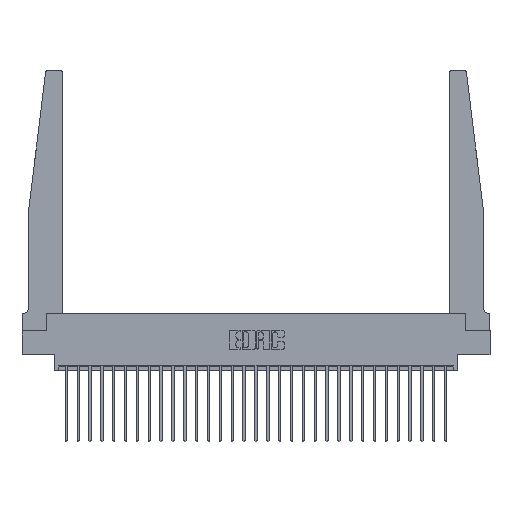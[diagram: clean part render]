
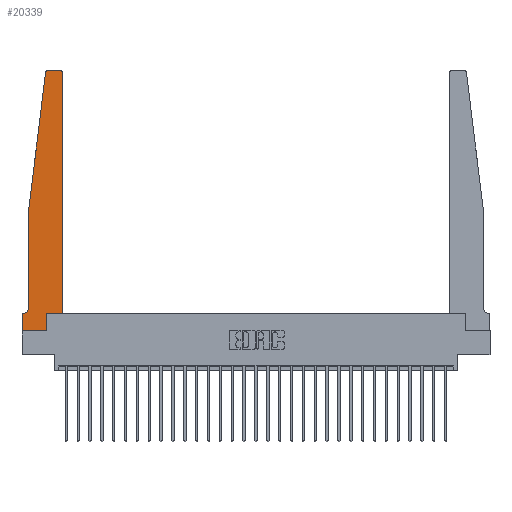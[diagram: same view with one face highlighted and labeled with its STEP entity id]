
A CAD part, top view. The second image highlights one B-rep face of the part: STEP entity #20339.
In plain terms, the highlighted planar face has unit normal (0, 0, 1).
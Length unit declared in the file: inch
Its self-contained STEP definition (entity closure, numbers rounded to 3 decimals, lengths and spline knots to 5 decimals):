
#234 = CIRCLE ( 'NONE', #23782, 0.03 ) ;
#404 = VECTOR ( 'NONE', #4082, 39.37008 ) ;
#507 = EDGE_CURVE ( 'NONE', #5747, #3042, #14602, .T. ) ;
#906 = FACE_OUTER_BOUND ( 'NONE', #13139, .T. ) ;
#1061 = CARTESIAN_POINT ( 'NONE',  ( 0.425, 0.18, 0.37 ) ) ;
#1441 = ORIENTED_EDGE ( 'NONE', *, *, #15282, .T. ) ;
#1762 = CARTESIAN_POINT ( 'NONE',  ( 0.065, 0.1875, 0.37 ) ) ;
#1978 = DIRECTION ( 'NONE',  ( 1., 0., 0. ) ) ;
#2156 = VERTEX_POINT ( 'NONE', #20838 ) ;
#2209 = CARTESIAN_POINT ( 'NONE',  ( 0.065, 1.25, 0.37 ) ) ;
#2315 = CARTESIAN_POINT ( 'NONE',  ( 0.27653, 2.75, 0.37 ) ) ;
#2370 = VECTOR ( 'NONE', #26618, 39.37008 ) ;
#3042 = VERTEX_POINT ( 'NONE', #2209 ) ;
#3288 = DIRECTION ( 'NONE',  ( 1., 0., 0. ) ) ;
#3348 = ORIENTED_EDGE ( 'NONE', *, *, #8446, .T. ) ;
#3850 = EDGE_CURVE ( 'NONE', #26175, #23514, #15615, .T. ) ;
#4082 = DIRECTION ( 'NONE',  ( 0., -1., 0. ) ) ;
#4130 = ORIENTED_EDGE ( 'NONE', *, *, #21587, .T. ) ;
#4142 = ORIENTED_EDGE ( 'NONE', *, *, #20375, .T. ) ;
#4181 = CARTESIAN_POINT ( 'NONE',  ( 0.425, 0.18, 0.37 ) ) ;
#4311 = DIRECTION ( 'NONE',  ( 0., 0., 1. ) ) ;
#4421 = EDGE_CURVE ( 'NONE', #25333, #2156, #17878, .T. ) ;
#4453 = VECTOR ( 'NONE', #3288, 39.37008 ) ;
#4528 = EDGE_CURVE ( 'NONE', #6403, #26307, #13869, .T. ) ;
#4544 = VECTOR ( 'NONE', #21095, 39.37008 ) ;
#5213 = LINE ( 'NONE', #1762, #4544 ) ;
#5747 = VERTEX_POINT ( 'NONE', #16254 ) ;
#5993 = CARTESIAN_POINT ( 'NONE',  ( 0.27653, 2.72, 0.37 ) ) ;
#6301 = PLANE ( 'NONE',  #25202 ) ;
#6403 = VERTEX_POINT ( 'NONE', #12019 ) ;
#6507 = CARTESIAN_POINT ( 'NONE',  ( 0.065, 1.25, 0.37 ) ) ;
#7302 = CARTESIAN_POINT ( 'NONE',  ( 0.015, 0.2375, 0.37 ) ) ;
#7697 = AXIS2_PLACEMENT_3D ( 'NONE', #5993, #20919, #8181 ) ;
#7716 = ORIENTED_EDGE ( 'NONE', *, *, #9852, .T. ) ;
#8181 = DIRECTION ( 'NONE',  ( 1., 0., 0. ) ) ;
#8446 = EDGE_CURVE ( 'NONE', #26307, #21052, #19672, .T. ) ;
#8549 = CARTESIAN_POINT ( 'NONE',  ( 0.065, 0.2375, 0.37 ) ) ;
#8960 = VERTEX_POINT ( 'NONE', #11787 ) ;
#9503 = DIRECTION ( 'NONE',  ( -1., 0., 0. ) ) ;
#9852 = EDGE_CURVE ( 'NONE', #8960, #6403, #15337, .T. ) ;
#10684 = LINE ( 'NONE', #6507, #15708 ) ;
#11787 = CARTESIAN_POINT ( 'NONE',  ( 0.2605, 0., 0.37 ) ) ;
#11877 = CARTESIAN_POINT ( 'NONE',  ( 0.25, 2.75, 0.37 ) ) ;
#12019 = CARTESIAN_POINT ( 'NONE',  ( 0.2605, 0.18, 0.37 ) ) ;
#12422 = LINE ( 'NONE', #19754, #22961 ) ;
#12840 = VERTEX_POINT ( 'NONE', #15918 ) ;
#13139 = EDGE_LOOP ( 'NONE', ( #15616, #15543, #19134, #22632, #21624, #25137, #1441, #4130, #7716, #15820, #3348, #4142 ) ) ;
#13349 = AXIS2_PLACEMENT_3D ( 'NONE', #7302, #22179, #9503 ) ;
#13619 = CARTESIAN_POINT ( 'NONE',  ( 0.425, 2.72, 0.37 ) ) ;
#13798 = EDGE_CURVE ( 'NONE', #23514, #5747, #17428, .T. ) ;
#13869 = LINE ( 'NONE', #1061, #4453 ) ;
#14060 = CARTESIAN_POINT ( 'NONE',  ( 0.425, 0.18, 0.37 ) ) ;
#14070 = VECTOR ( 'NONE', #16195, 39.37008 ) ;
#14602 = LINE ( 'NONE', #20191, #2370 ) ;
#14981 = DIRECTION ( 'NONE',  ( 0., 0., 1. ) ) ;
#15282 = EDGE_CURVE ( 'NONE', #21205, #12840, #22570, .T. ) ;
#15337 = LINE ( 'NONE', #20626, #25832 ) ;
#15543 = ORIENTED_EDGE ( 'NONE', *, *, #13798, .T. ) ;
#15615 = LINE ( 'NONE', #11877, #26100 ) ;
#15616 = ORIENTED_EDGE ( 'NONE', *, *, #3850, .T. ) ;
#15708 = VECTOR ( 'NONE', #23497, 39.37008 ) ;
#15820 = ORIENTED_EDGE ( 'NONE', *, *, #4528, .T. ) ;
#15918 = CARTESIAN_POINT ( 'NONE',  ( 0., 0., 0.37 ) ) ;
#16195 = DIRECTION ( 'NONE',  ( 0., 1., 0. ) ) ;
#16254 = CARTESIAN_POINT ( 'NONE',  ( 0.24675, 2.72367, 0.37 ) ) ;
#16610 = CARTESIAN_POINT ( 'NONE',  ( 0.395, 2.75, 0.37 ) ) ;
#16684 = EDGE_CURVE ( 'NONE', #3042, #25333, #10684, .T. ) ;
#17190 = CARTESIAN_POINT ( 'NONE',  ( 0.395, 2.72, 0.37 ) ) ;
#17428 = CIRCLE ( 'NONE', #7697, 0.03 ) ;
#17878 = CIRCLE ( 'NONE', #13349, 0.05 ) ;
#18586 = CARTESIAN_POINT ( 'NONE',  ( 0., 0.1875, 0.37 ) ) ;
#19069 = CARTESIAN_POINT ( 'NONE',  ( 0., 0., 0.37 ) ) ;
#19134 = ORIENTED_EDGE ( 'NONE', *, *, #507, .T. ) ;
#19287 = DIRECTION ( 'NONE',  ( 1., 0., 0. ) ) ;
#19672 = LINE ( 'NONE', #14060, #14070 ) ;
#19754 = CARTESIAN_POINT ( 'NONE',  ( 0., 0., 0.37 ) ) ;
#20191 = CARTESIAN_POINT ( 'NONE',  ( 0.065, 1.25, 0.37 ) ) ;
#20339 = ADVANCED_FACE ( 'NONE', ( #906 ), #6301, .T. ) ;
#20375 = EDGE_CURVE ( 'NONE', #21052, #26175, #234, .T. ) ;
#20626 = CARTESIAN_POINT ( 'NONE',  ( 0.2605, 0.18, 0.37 ) ) ;
#20838 = CARTESIAN_POINT ( 'NONE',  ( 0.015, 0.1875, 0.37 ) ) ;
#20919 = DIRECTION ( 'NONE',  ( 0., 0., 1. ) ) ;
#21052 = VERTEX_POINT ( 'NONE', #13619 ) ;
#21095 = DIRECTION ( 'NONE',  ( -1., 0., 0. ) ) ;
#21205 = VERTEX_POINT ( 'NONE', #18586 ) ;
#21587 = EDGE_CURVE ( 'NONE', #12840, #8960, #12422, .T. ) ;
#21624 = ORIENTED_EDGE ( 'NONE', *, *, #4421, .T. ) ;
#21872 = DIRECTION ( 'NONE',  ( 1., 0., 0. ) ) ;
#22179 = DIRECTION ( 'NONE',  ( 0., 0., -1. ) ) ;
#22570 = LINE ( 'NONE', #19069, #404 ) ;
#22632 = ORIENTED_EDGE ( 'NONE', *, *, #16684, .T. ) ;
#22723 = DIRECTION ( 'NONE',  ( 0., 1., 0. ) ) ;
#22961 = VECTOR ( 'NONE', #21872, 39.37008 ) ;
#23497 = DIRECTION ( 'NONE',  ( 0., -1., 0. ) ) ;
#23514 = VERTEX_POINT ( 'NONE', #2315 ) ;
#23782 = AXIS2_PLACEMENT_3D ( 'NONE', #17190, #4311, #19287 ) ;
#25137 = ORIENTED_EDGE ( 'NONE', *, *, #26266, .T. ) ;
#25202 = AXIS2_PLACEMENT_3D ( 'NONE', #27543, #14981, #1978 ) ;
#25333 = VERTEX_POINT ( 'NONE', #8549 ) ;
#25832 = VECTOR ( 'NONE', #22723, 39.37008 ) ;
#26100 = VECTOR ( 'NONE', #26621, 39.37008 ) ;
#26175 = VERTEX_POINT ( 'NONE', #16610 ) ;
#26266 = EDGE_CURVE ( 'NONE', #2156, #21205, #5213, .T. ) ;
#26307 = VERTEX_POINT ( 'NONE', #4181 ) ;
#26618 = DIRECTION ( 'NONE',  ( -0.122, -0.992, 0. ) ) ;
#26621 = DIRECTION ( 'NONE',  ( -1., 0., 0. ) ) ;
#27543 = CARTESIAN_POINT ( 'NONE',  ( 0., 0.1875, 0.37 ) ) ;
